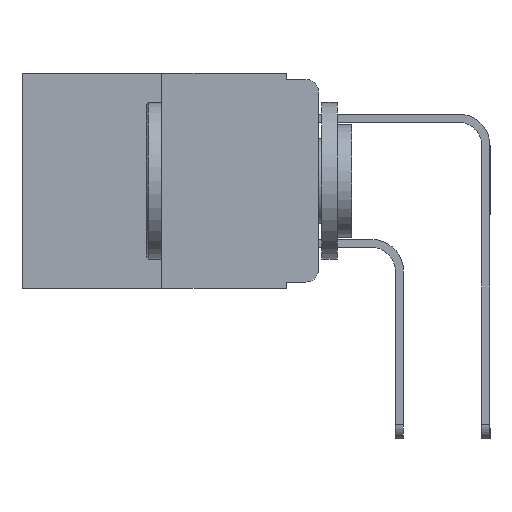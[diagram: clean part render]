
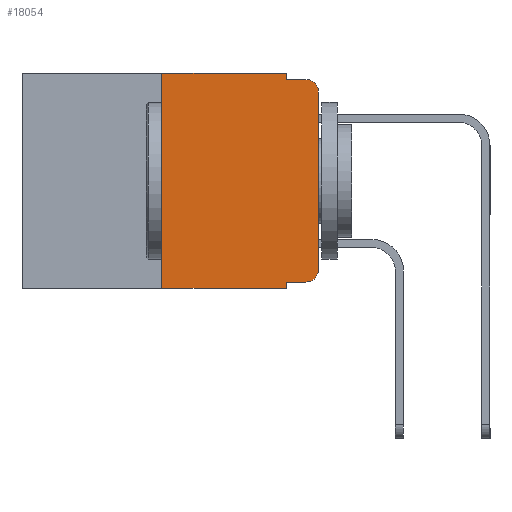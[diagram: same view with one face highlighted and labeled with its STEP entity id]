
A CAD part, left-side view. The second image highlights one B-rep face of the part: STEP entity #18054.
In plain terms, the highlighted planar face has unit normal (-1, 0, 0).
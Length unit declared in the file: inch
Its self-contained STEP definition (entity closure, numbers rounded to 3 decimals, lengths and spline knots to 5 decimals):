
#49 = LINE ( 'NONE', #18624, #4659 ) ;
#253 = CARTESIAN_POINT ( 'NONE',  ( 0., 0.051, 0. ) ) ;
#291 = ORIENTED_EDGE ( 'NONE', *, *, #17975, .F. ) ;
#327 = ORIENTED_EDGE ( 'NONE', *, *, #5919, .T. ) ;
#392 = DIRECTION ( 'NONE',  ( -1., 0., 0. ) ) ;
#534 = VERTEX_POINT ( 'NONE', #8444 ) ;
#911 = CARTESIAN_POINT ( 'NONE',  ( 0., 0.25, 0. ) ) ;
#1001 = ORIENTED_EDGE ( 'NONE', *, *, #16494, .T. ) ;
#1434 = DIRECTION ( 'NONE',  ( 0., 0., -1. ) ) ;
#1997 = AXIS2_PLACEMENT_3D ( 'NONE', #5510, #19069, #7452 ) ;
#2247 = VERTEX_POINT ( 'NONE', #15531 ) ;
#3054 = VERTEX_POINT ( 'NONE', #12532 ) ;
#3101 = CARTESIAN_POINT ( 'NONE',  ( 0., 0.051, -0.333 ) ) ;
#4012 = CARTESIAN_POINT ( 'NONE',  ( 0., 0.473, 0. ) ) ;
#4452 = EDGE_CURVE ( 'NONE', #18625, #534, #15805, .T. ) ;
#4659 = VECTOR ( 'NONE', #20513, 39.37008 ) ;
#4847 = LINE ( 'NONE', #253, #9388 ) ;
#4946 = EDGE_CURVE ( 'NONE', #18625, #22765, #4847, .T. ) ;
#5318 = LINE ( 'NONE', #24171, #10495 ) ;
#5503 = VERTEX_POINT ( 'NONE', #19820 ) ;
#5510 = CARTESIAN_POINT ( 'NONE',  ( 0., 0.02, -0.03 ) ) ;
#5919 = EDGE_CURVE ( 'NONE', #5503, #13735, #13909, .T. ) ;
#6058 = VECTOR ( 'NONE', #21989, 39.37008 ) ;
#6348 = VERTEX_POINT ( 'NONE', #911 ) ;
#6380 = LINE ( 'NONE', #4012, #14815 ) ;
#7452 = DIRECTION ( 'NONE',  ( 0., 0., -1. ) ) ;
#7825 = EDGE_LOOP ( 'NONE', ( #1001, #327, #291, #13720, #13513, #13274, #12960, #12921, #12116, #11661 ) ) ;
#8245 = DIRECTION ( 'NONE',  ( 0., 0., 1. ) ) ;
#8444 = CARTESIAN_POINT ( 'NONE',  ( 0., 0.02, -0.333 ) ) ;
#8543 = CARTESIAN_POINT ( 'NONE',  ( 0., 0.051, -0.333 ) ) ;
#8589 = DIRECTION ( 'NONE',  ( 0., -1., 0. ) ) ;
#8883 = VERTEX_POINT ( 'NONE', #22490 ) ;
#8945 = CARTESIAN_POINT ( 'NONE',  ( 0., 0.051, -0.343 ) ) ;
#9388 = VECTOR ( 'NONE', #21475, 39.37008 ) ;
#9781 = VECTOR ( 'NONE', #8589, 39.37008 ) ;
#10118 = CARTESIAN_POINT ( 'NONE',  ( 0., 0., 0. ) ) ;
#10495 = VECTOR ( 'NONE', #18549, 39.37008 ) ;
#11540 = CARTESIAN_POINT ( 'NONE',  ( 0., 0.02, -0.01 ) ) ;
#11661 = ORIENTED_EDGE ( 'NONE', *, *, #24664, .T. ) ;
#12109 = CARTESIAN_POINT ( 'NONE',  ( 0., 0.02, -0.313 ) ) ;
#12116 = ORIENTED_EDGE ( 'NONE', *, *, #4452, .T. ) ;
#12532 = CARTESIAN_POINT ( 'NONE',  ( 0., 0.051, 0. ) ) ;
#12921 = ORIENTED_EDGE ( 'NONE', *, *, #4946, .F. ) ;
#12960 = ORIENTED_EDGE ( 'NONE', *, *, #20403, .T. ) ;
#13076 = DIRECTION ( 'NONE',  ( 1., 0., 0. ) ) ;
#13274 = ORIENTED_EDGE ( 'NONE', *, *, #18269, .F. ) ;
#13513 = ORIENTED_EDGE ( 'NONE', *, *, #16376, .F. ) ;
#13682 = CIRCLE ( 'NONE', #16154, 0.02 ) ;
#13717 = VECTOR ( 'NONE', #8245, 39.37008 ) ;
#13720 = ORIENTED_EDGE ( 'NONE', *, *, #19997, .F. ) ;
#13735 = VERTEX_POINT ( 'NONE', #11540 ) ;
#13909 = CIRCLE ( 'NONE', #1997, 0.02 ) ;
#14071 = DIRECTION ( 'NONE',  ( 0., 0., -1. ) ) ;
#14166 = LINE ( 'NONE', #24874, #23620 ) ;
#14815 = VECTOR ( 'NONE', #17601, 39.37008 ) ;
#14888 = CARTESIAN_POINT ( 'NONE',  ( 0., 0., -0.313 ) ) ;
#14968 = PLANE ( 'NONE',  #15558 ) ;
#15342 = VERTEX_POINT ( 'NONE', #14888 ) ;
#15531 = CARTESIAN_POINT ( 'NONE',  ( 0., 0.25, -0.343 ) ) ;
#15558 = AXIS2_PLACEMENT_3D ( 'NONE', #24415, #13076, #1434 ) ;
#15805 = LINE ( 'NONE', #8543, #6058 ) ;
#16154 = AXIS2_PLACEMENT_3D ( 'NONE', #12109, #392, #14071 ) ;
#16196 = LINE ( 'NONE', #18267, #9781 ) ;
#16376 = EDGE_CURVE ( 'NONE', #6348, #3054, #6380, .T. ) ;
#16494 = EDGE_CURVE ( 'NONE', #15342, #5503, #17039, .T. ) ;
#17039 = LINE ( 'NONE', #10118, #13717 ) ;
#17601 = DIRECTION ( 'NONE',  ( 0., -1., 0. ) ) ;
#17975 = EDGE_CURVE ( 'NONE', #8883, #13735, #5318, .T. ) ;
#18054 = ADVANCED_FACE ( 'NONE', ( #18370 ), #14968, .F. ) ;
#18267 = CARTESIAN_POINT ( 'NONE',  ( 0., 0.473, -0.343 ) ) ;
#18269 = EDGE_CURVE ( 'NONE', #2247, #6348, #14166, .T. ) ;
#18370 = FACE_OUTER_BOUND ( 'NONE', #7825, .T. ) ;
#18549 = DIRECTION ( 'NONE',  ( 0., -1., 0. ) ) ;
#18624 = CARTESIAN_POINT ( 'NONE',  ( 0., 0.051, 0. ) ) ;
#18625 = VERTEX_POINT ( 'NONE', #3101 ) ;
#19069 = DIRECTION ( 'NONE',  ( -1., 0., 0. ) ) ;
#19438 = DIRECTION ( 'NONE',  ( 0., 0., 1. ) ) ;
#19820 = CARTESIAN_POINT ( 'NONE',  ( 0., 0., -0.03 ) ) ;
#19997 = EDGE_CURVE ( 'NONE', #3054, #8883, #49, .T. ) ;
#20403 = EDGE_CURVE ( 'NONE', #2247, #22765, #16196, .T. ) ;
#20513 = DIRECTION ( 'NONE',  ( 0., 0., -1. ) ) ;
#21475 = DIRECTION ( 'NONE',  ( 0., 0., -1. ) ) ;
#21989 = DIRECTION ( 'NONE',  ( 0., -1., 0. ) ) ;
#22490 = CARTESIAN_POINT ( 'NONE',  ( 0., 0.051, -0.01 ) ) ;
#22765 = VERTEX_POINT ( 'NONE', #8945 ) ;
#23620 = VECTOR ( 'NONE', #19438, 39.37008 ) ;
#24171 = CARTESIAN_POINT ( 'NONE',  ( 0., 0.051, -0.01 ) ) ;
#24415 = CARTESIAN_POINT ( 'NONE',  ( 0., 0.473, 0. ) ) ;
#24664 = EDGE_CURVE ( 'NONE', #534, #15342, #13682, .T. ) ;
#24874 = CARTESIAN_POINT ( 'NONE',  ( 0., 0.25, 0. ) ) ;
